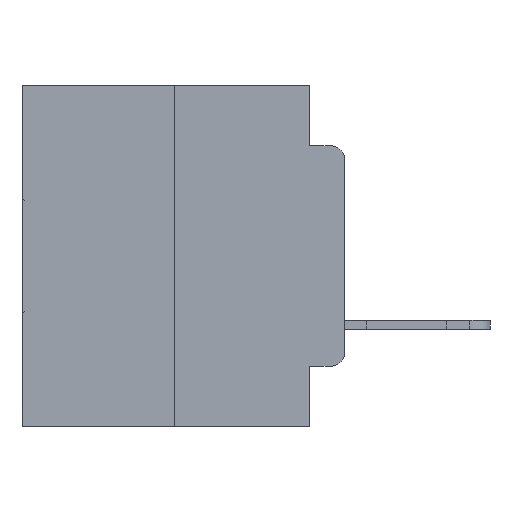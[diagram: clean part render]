
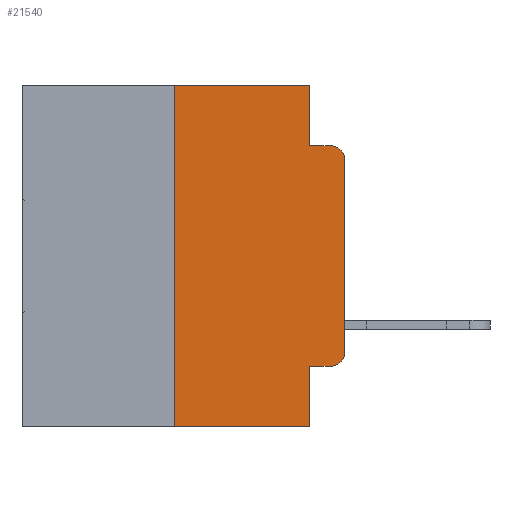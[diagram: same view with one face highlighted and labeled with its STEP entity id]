
A CAD part, left-side view. The second image highlights one B-rep face of the part: STEP entity #21540.
In plain terms, the highlighted planar face has unit normal (-1, 0, 0).
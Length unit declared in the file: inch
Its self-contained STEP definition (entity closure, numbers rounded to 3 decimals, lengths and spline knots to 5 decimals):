
#686 = CARTESIAN_POINT ( 'NONE',  ( 0., 0.473, -0.5 ) ) ;
#1514 = LINE ( 'NONE', #11711, #7798 ) ;
#2414 = VECTOR ( 'NONE', #25364, 39.37008 ) ;
#2600 = AXIS2_PLACEMENT_3D ( 'NONE', #29241, #27202, #13942 ) ;
#2970 = CARTESIAN_POINT ( 'NONE',  ( 0., 0.051, 0. ) ) ;
#3489 = DIRECTION ( 'NONE',  ( 0., -1., 0. ) ) ;
#3853 = CARTESIAN_POINT ( 'NONE',  ( 0., 0., -0.3915 ) ) ;
#3900 = CARTESIAN_POINT ( 'NONE',  ( 0., 0.02, -0.0885 ) ) ;
#4406 = CARTESIAN_POINT ( 'NONE',  ( 0., 0.051, 0. ) ) ;
#5125 = AXIS2_PLACEMENT_3D ( 'NONE', #24796, #11094, #26921 ) ;
#5239 = LINE ( 'NONE', #6205, #29159 ) ;
#5467 = LINE ( 'NONE', #26910, #28661 ) ;
#5689 = DIRECTION ( 'NONE',  ( 0., 0., -1. ) ) ;
#6041 = DIRECTION ( 'NONE',  ( 0., 0., 1. ) ) ;
#6205 = CARTESIAN_POINT ( 'NONE',  ( 0., 0.473, 0. ) ) ;
#6304 = PLANE ( 'NONE',  #2600 ) ;
#6316 = CARTESIAN_POINT ( 'NONE',  ( 0., 0.051, -0.5 ) ) ;
#6537 = CARTESIAN_POINT ( 'NONE',  ( 0., 0.25, 0. ) ) ;
#6788 = VERTEX_POINT ( 'NONE', #14399 ) ;
#7097 = ORIENTED_EDGE ( 'NONE', *, *, #27376, .F. ) ;
#7469 = ORIENTED_EDGE ( 'NONE', *, *, #8549, .F. ) ;
#7798 = VECTOR ( 'NONE', #29555, 39.37008 ) ;
#8099 = VECTOR ( 'NONE', #25271, 39.37008 ) ;
#8549 = EDGE_CURVE ( 'NONE', #22277, #19959, #1514, .T. ) ;
#9483 = ORIENTED_EDGE ( 'NONE', *, *, #11916, .T. ) ;
#10357 = ORIENTED_EDGE ( 'NONE', *, *, #17376, .T. ) ;
#10882 = VERTEX_POINT ( 'NONE', #29464 ) ;
#10951 = VECTOR ( 'NONE', #5689, 39.37008 ) ;
#11094 = DIRECTION ( 'NONE',  ( -1., 0., 0. ) ) ;
#11587 = VERTEX_POINT ( 'NONE', #4406 ) ;
#11711 = CARTESIAN_POINT ( 'NONE',  ( 0., 0.051, -0.0885 ) ) ;
#11916 = EDGE_CURVE ( 'NONE', #28801, #19959, #29244, .T. ) ;
#12049 = DIRECTION ( 'NONE',  ( 0., -1., 0. ) ) ;
#12327 = EDGE_LOOP ( 'NONE', ( #29931, #9483, #7469, #22300, #7097, #21635, #30628, #23360, #10357, #15017 ) ) ;
#13051 = CARTESIAN_POINT ( 'NONE',  ( 0., 0.02, -0.3915 ) ) ;
#13909 = CARTESIAN_POINT ( 'NONE',  ( 0., 0.051, -0.4115 ) ) ;
#13919 = CARTESIAN_POINT ( 'NONE',  ( 0., 0.051, -0.0885 ) ) ;
#13942 = DIRECTION ( 'NONE',  ( 0., 0., -1. ) ) ;
#14196 = EDGE_CURVE ( 'NONE', #25460, #16104, #27918, .T. ) ;
#14399 = CARTESIAN_POINT ( 'NONE',  ( 0., 0.25, -0.5 ) ) ;
#14633 = CARTESIAN_POINT ( 'NONE',  ( 0., 0.051, -0.4115 ) ) ;
#14749 = LINE ( 'NONE', #6537, #8099 ) ;
#15017 = ORIENTED_EDGE ( 'NONE', *, *, #14196, .T. ) ;
#15259 = LINE ( 'NONE', #18843, #2414 ) ;
#15441 = VERTEX_POINT ( 'NONE', #13909 ) ;
#15506 = DIRECTION ( 'NONE',  ( 0., 0., -1. ) ) ;
#16104 = VERTEX_POINT ( 'NONE', #3853 ) ;
#16571 = CARTESIAN_POINT ( 'NONE',  ( 0., 0.02, -0.4115 ) ) ;
#17028 = EDGE_CURVE ( 'NONE', #6788, #27428, #24483, .T. ) ;
#17376 = EDGE_CURVE ( 'NONE', #15441, #25460, #23422, .T. ) ;
#17645 = VECTOR ( 'NONE', #12049, 39.37008 ) ;
#18421 = DIRECTION ( 'NONE',  ( 0., -1., 0. ) ) ;
#18698 = VECTOR ( 'NONE', #18421, 39.37008 ) ;
#18843 = CARTESIAN_POINT ( 'NONE',  ( 0., 0.051, 0. ) ) ;
#19775 = EDGE_CURVE ( 'NONE', #16104, #28801, #5467, .T. ) ;
#19959 = VERTEX_POINT ( 'NONE', #3900 ) ;
#21514 = AXIS2_PLACEMENT_3D ( 'NONE', #13051, #28567, #15506 ) ;
#21540 = ADVANCED_FACE ( 'NONE', ( #22671 ), #6304, .F. ) ;
#21635 = ORIENTED_EDGE ( 'NONE', *, *, #27499, .F. ) ;
#22277 = VERTEX_POINT ( 'NONE', #13919 ) ;
#22300 = ORIENTED_EDGE ( 'NONE', *, *, #30315, .F. ) ;
#22671 = FACE_OUTER_BOUND ( 'NONE', #12327, .T. ) ;
#23201 = LINE ( 'NONE', #2970, #10951 ) ;
#23360 = ORIENTED_EDGE ( 'NONE', *, *, #24693, .F. ) ;
#23422 = LINE ( 'NONE', #14633, #17645 ) ;
#24194 = CARTESIAN_POINT ( 'NONE',  ( 0., 0., -0.1085 ) ) ;
#24483 = LINE ( 'NONE', #686, #18698 ) ;
#24693 = EDGE_CURVE ( 'NONE', #15441, #27428, #15259, .T. ) ;
#24796 = CARTESIAN_POINT ( 'NONE',  ( 0., 0.02, -0.1085 ) ) ;
#25271 = DIRECTION ( 'NONE',  ( 0., 0., 1. ) ) ;
#25364 = DIRECTION ( 'NONE',  ( 0., 0., -1. ) ) ;
#25460 = VERTEX_POINT ( 'NONE', #16571 ) ;
#26910 = CARTESIAN_POINT ( 'NONE',  ( 0., 0., 0. ) ) ;
#26921 = DIRECTION ( 'NONE',  ( 0., 0., -1. ) ) ;
#27202 = DIRECTION ( 'NONE',  ( 1., 0., 0. ) ) ;
#27376 = EDGE_CURVE ( 'NONE', #10882, #11587, #5239, .T. ) ;
#27428 = VERTEX_POINT ( 'NONE', #6316 ) ;
#27499 = EDGE_CURVE ( 'NONE', #6788, #10882, #14749, .T. ) ;
#27918 = CIRCLE ( 'NONE', #21514, 0.02 ) ;
#28567 = DIRECTION ( 'NONE',  ( -1., 0., 0. ) ) ;
#28661 = VECTOR ( 'NONE', #6041, 39.37008 ) ;
#28801 = VERTEX_POINT ( 'NONE', #24194 ) ;
#29159 = VECTOR ( 'NONE', #3489, 39.37008 ) ;
#29241 = CARTESIAN_POINT ( 'NONE',  ( 0., 0.473, 0. ) ) ;
#29244 = CIRCLE ( 'NONE', #5125, 0.02 ) ;
#29464 = CARTESIAN_POINT ( 'NONE',  ( 0., 0.25, 0. ) ) ;
#29555 = DIRECTION ( 'NONE',  ( 0., -1., 0. ) ) ;
#29931 = ORIENTED_EDGE ( 'NONE', *, *, #19775, .T. ) ;
#30315 = EDGE_CURVE ( 'NONE', #11587, #22277, #23201, .T. ) ;
#30628 = ORIENTED_EDGE ( 'NONE', *, *, #17028, .T. ) ;
